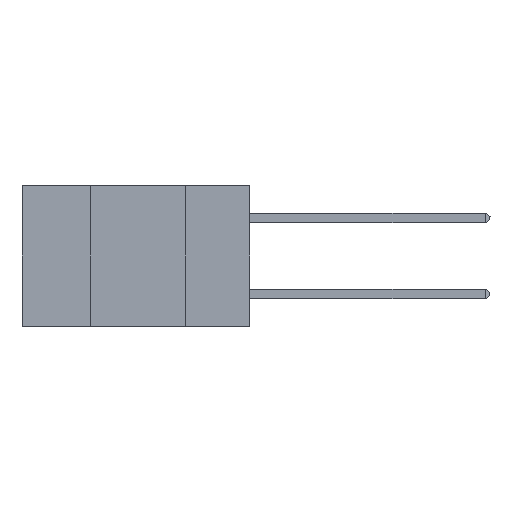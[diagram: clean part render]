
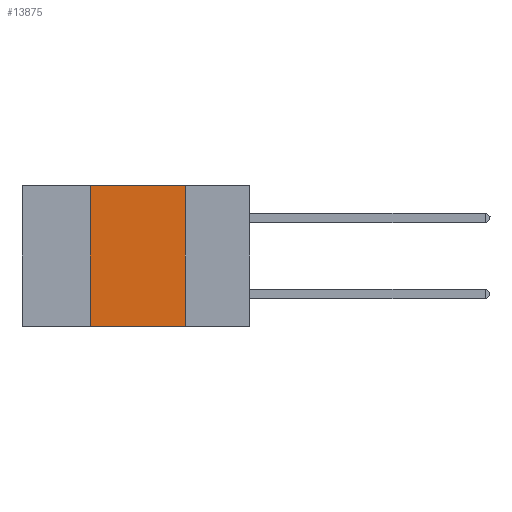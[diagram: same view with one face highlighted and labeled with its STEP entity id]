
A CAD part, left-side view. The second image highlights one B-rep face of the part: STEP entity #13875.
In plain terms, the highlighted planar face has unit normal (-1, 0, 0).
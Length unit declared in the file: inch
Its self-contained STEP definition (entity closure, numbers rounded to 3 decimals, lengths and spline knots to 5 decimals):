
#1601 = VERTEX_POINT ( 'NONE', #13703 ) ;
#1797 = DIRECTION ( 'NONE',  ( 0., -1., 0. ) ) ;
#2214 = FACE_OUTER_BOUND ( 'NONE', #14728, .T. ) ;
#2440 = ORIENTED_EDGE ( 'NONE', *, *, #24206, .F. ) ;
#4125 = LINE ( 'NONE', #15339, #21287 ) ;
#5914 = DIRECTION ( 'NONE',  ( 1., 0., 0. ) ) ;
#6632 = CARTESIAN_POINT ( 'NONE',  ( 0., 0.17, 0. ) ) ;
#6947 = VECTOR ( 'NONE', #1797, 39.37008 ) ;
#8611 = VECTOR ( 'NONE', #22825, 39.37008 ) ;
#9259 = LINE ( 'NONE', #23485, #6947 ) ;
#10419 = LINE ( 'NONE', #6632, #18996 ) ;
#10750 = ORIENTED_EDGE ( 'NONE', *, *, #46467, .F. ) ;
#12901 = CARTESIAN_POINT ( 'NONE',  ( 0., 0.42, 0. ) ) ;
#13703 = CARTESIAN_POINT ( 'NONE',  ( 0., 0.17, 0. ) ) ;
#13875 = ADVANCED_FACE ( 'NONE', ( #2214 ), #46047, .F. ) ;
#14446 = ORIENTED_EDGE ( 'NONE', *, *, #26594, .T. ) ;
#14728 = EDGE_LOOP ( 'NONE', ( #2440, #40061, #10750, #14446 ) ) ;
#15339 = CARTESIAN_POINT ( 'NONE',  ( 0., 0.42, 0. ) ) ;
#18329 = LINE ( 'NONE', #19147, #8611 ) ;
#18917 = EDGE_CURVE ( 'NONE', #22072, #1601, #18329, .T. ) ;
#18996 = VECTOR ( 'NONE', #25007, 39.37008 ) ;
#19147 = CARTESIAN_POINT ( 'NONE',  ( 0., 0.6, 0. ) ) ;
#20474 = CARTESIAN_POINT ( 'NONE',  ( 0., 0.6, 0. ) ) ;
#21287 = VECTOR ( 'NONE', #44613, 39.37008 ) ;
#22072 = VERTEX_POINT ( 'NONE', #12901 ) ;
#22825 = DIRECTION ( 'NONE',  ( 0., -1., 0. ) ) ;
#23485 = CARTESIAN_POINT ( 'NONE',  ( 0., 0.6, -0.37 ) ) ;
#24206 = EDGE_CURVE ( 'NONE', #1601, #46951, #10419, .T. ) ;
#24970 = AXIS2_PLACEMENT_3D ( 'NONE', #20474, #5914, #31503 ) ;
#25007 = DIRECTION ( 'NONE',  ( 0., 0., -1. ) ) ;
#26594 = EDGE_CURVE ( 'NONE', #45925, #46951, #9259, .T. ) ;
#27200 = CARTESIAN_POINT ( 'NONE',  ( 0., 0.42, -0.37 ) ) ;
#31503 = DIRECTION ( 'NONE',  ( 0., 0., -1. ) ) ;
#40061 = ORIENTED_EDGE ( 'NONE', *, *, #18917, .F. ) ;
#44613 = DIRECTION ( 'NONE',  ( 0., 0., 1. ) ) ;
#45925 = VERTEX_POINT ( 'NONE', #27200 ) ;
#46047 = PLANE ( 'NONE',  #24970 ) ;
#46467 = EDGE_CURVE ( 'NONE', #45925, #22072, #4125, .T. ) ;
#46951 = VERTEX_POINT ( 'NONE', #47275 ) ;
#47275 = CARTESIAN_POINT ( 'NONE',  ( 0., 0.17, -0.37 ) ) ;
